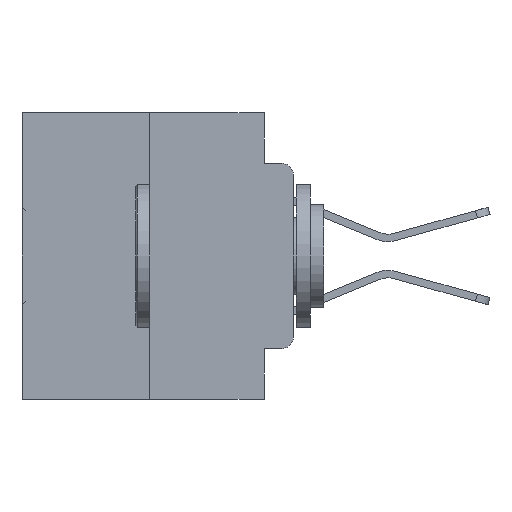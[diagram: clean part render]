
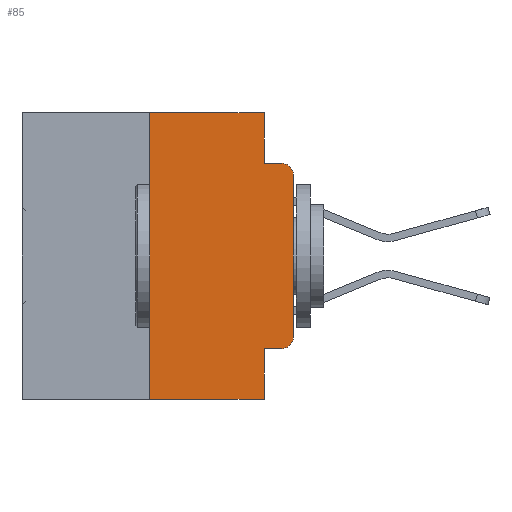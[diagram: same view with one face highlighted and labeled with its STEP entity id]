
A CAD part, left-side view. The second image highlights one B-rep face of the part: STEP entity #85.
In plain terms, the highlighted planar face has unit normal (-1, 0, 0).
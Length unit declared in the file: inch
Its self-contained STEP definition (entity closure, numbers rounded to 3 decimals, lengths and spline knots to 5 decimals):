
#85 = ADVANCED_FACE ( 'NONE', ( #22199 ), #4309, .F. ) ;
#927 = CARTESIAN_POINT ( 'NONE',  ( 0., 0.051, -0.5 ) ) ;
#1116 = AXIS2_PLACEMENT_3D ( 'NONE', #32327, #17435, #2145 ) ;
#1178 = LINE ( 'NONE', #29608, #19971 ) ;
#1871 = DIRECTION ( 'NONE',  ( 0., 0., -1. ) ) ;
#2145 = DIRECTION ( 'NONE',  ( 0., 0., -1. ) ) ;
#2668 = VECTOR ( 'NONE', #17198, 39.37008 ) ;
#2697 = ORIENTED_EDGE ( 'NONE', *, *, #23551, .T. ) ;
#4086 = CARTESIAN_POINT ( 'NONE',  ( 0., 0.473, -0.5 ) ) ;
#4309 = PLANE ( 'NONE',  #28458 ) ;
#4432 = LINE ( 'NONE', #19860, #9673 ) ;
#4903 = EDGE_CURVE ( 'NONE', #10895, #21757, #29985, .T. ) ;
#5461 = VECTOR ( 'NONE', #10900, 39.37008 ) ;
#5634 = CARTESIAN_POINT ( 'NONE',  ( 0., 0.051, -0.4115 ) ) ;
#6263 = LINE ( 'NONE', #5634, #5461 ) ;
#6623 = EDGE_CURVE ( 'NONE', #12689, #10895, #6263, .T. ) ;
#6756 = VECTOR ( 'NONE', #13030, 39.37008 ) ;
#6823 = CIRCLE ( 'NONE', #1116, 0.02 ) ;
#7891 = LINE ( 'NONE', #4086, #14583 ) ;
#8560 = VERTEX_POINT ( 'NONE', #927 ) ;
#8759 = LINE ( 'NONE', #29683, #2668 ) ;
#9404 = DIRECTION ( 'NONE',  ( 0., -1., 0. ) ) ;
#9613 = DIRECTION ( 'NONE',  ( 0., 0., -1. ) ) ;
#9673 = VECTOR ( 'NONE', #9613, 39.37008 ) ;
#9747 = CARTESIAN_POINT ( 'NONE',  ( 0., 0.473, 0. ) ) ;
#10529 = CARTESIAN_POINT ( 'NONE',  ( 0., 0.25, 0. ) ) ;
#10895 = VERTEX_POINT ( 'NONE', #31496 ) ;
#10900 = DIRECTION ( 'NONE',  ( 0., -1., 0. ) ) ;
#10946 = CARTESIAN_POINT ( 'NONE',  ( 0., 0.25, 0. ) ) ;
#11405 = CARTESIAN_POINT ( 'NONE',  ( 0., 0.051, -0.0885 ) ) ;
#11745 = EDGE_CURVE ( 'NONE', #12689, #8560, #4432, .T. ) ;
#12689 = VERTEX_POINT ( 'NONE', #22904 ) ;
#13030 = DIRECTION ( 'NONE',  ( 0., 0., 1. ) ) ;
#13120 = ORIENTED_EDGE ( 'NONE', *, *, #15068, .F. ) ;
#13384 = EDGE_CURVE ( 'NONE', #21767, #18667, #13447, .T. ) ;
#13447 = LINE ( 'NONE', #10529, #6756 ) ;
#13586 = VERTEX_POINT ( 'NONE', #11405 ) ;
#14304 = DIRECTION ( 'NONE',  ( 0., -1., 0. ) ) ;
#14453 = CARTESIAN_POINT ( 'NONE',  ( 0., 0.473, 0. ) ) ;
#14583 = VECTOR ( 'NONE', #14304, 39.37008 ) ;
#15068 = EDGE_CURVE ( 'NONE', #31848, #13586, #1178, .T. ) ;
#15101 = ORIENTED_EDGE ( 'NONE', *, *, #11745, .F. ) ;
#15467 = ORIENTED_EDGE ( 'NONE', *, *, #17006, .F. ) ;
#16682 = ORIENTED_EDGE ( 'NONE', *, *, #6623, .T. ) ;
#16862 = CARTESIAN_POINT ( 'NONE',  ( 0., 0., -0.3915 ) ) ;
#17006 = EDGE_CURVE ( 'NONE', #18667, #31848, #23812, .T. ) ;
#17086 = VECTOR ( 'NONE', #24507, 39.37008 ) ;
#17162 = DIRECTION ( 'NONE',  ( -1., 0., 0. ) ) ;
#17198 = DIRECTION ( 'NONE',  ( 0., 0., 1. ) ) ;
#17435 = DIRECTION ( 'NONE',  ( -1., 0., 0. ) ) ;
#18483 = VERTEX_POINT ( 'NONE', #20222 ) ;
#18667 = VERTEX_POINT ( 'NONE', #10946 ) ;
#18933 = EDGE_CURVE ( 'NONE', #21767, #8560, #7891, .T. ) ;
#19454 = CARTESIAN_POINT ( 'NONE',  ( 0., 0.051, -0.0885 ) ) ;
#19860 = CARTESIAN_POINT ( 'NONE',  ( 0., 0.051, 0. ) ) ;
#19971 = VECTOR ( 'NONE', #22204, 39.37008 ) ;
#20198 = EDGE_CURVE ( 'NONE', #13586, #18483, #29416, .T. ) ;
#20222 = CARTESIAN_POINT ( 'NONE',  ( 0., 0.02, -0.0885 ) ) ;
#21263 = DIRECTION ( 'NONE',  ( 1., 0., 0. ) ) ;
#21757 = VERTEX_POINT ( 'NONE', #16862 ) ;
#21767 = VERTEX_POINT ( 'NONE', #31894 ) ;
#21792 = EDGE_LOOP ( 'NONE', ( #2697, #31109, #25737, #13120, #15467, #25358, #32656, #15101, #16682, #24210 ) ) ;
#21867 = EDGE_CURVE ( 'NONE', #28294, #18483, #6823, .T. ) ;
#22199 = FACE_OUTER_BOUND ( 'NONE', #21792, .T. ) ;
#22204 = DIRECTION ( 'NONE',  ( 0., 0., -1. ) ) ;
#22809 = VECTOR ( 'NONE', #9404, 39.37008 ) ;
#22904 = CARTESIAN_POINT ( 'NONE',  ( 0., 0.051, -0.4115 ) ) ;
#23551 = EDGE_CURVE ( 'NONE', #21757, #28294, #8759, .T. ) ;
#23812 = LINE ( 'NONE', #14453, #17086 ) ;
#24210 = ORIENTED_EDGE ( 'NONE', *, *, #4903, .T. ) ;
#24507 = DIRECTION ( 'NONE',  ( 0., -1., 0. ) ) ;
#25358 = ORIENTED_EDGE ( 'NONE', *, *, #13384, .F. ) ;
#25392 = CARTESIAN_POINT ( 'NONE',  ( 0., 0.051, 0. ) ) ;
#25737 = ORIENTED_EDGE ( 'NONE', *, *, #20198, .F. ) ;
#26678 = DIRECTION ( 'NONE',  ( 0., 0., -1. ) ) ;
#28294 = VERTEX_POINT ( 'NONE', #29577 ) ;
#28458 = AXIS2_PLACEMENT_3D ( 'NONE', #9747, #21263, #26678 ) ;
#29416 = LINE ( 'NONE', #19454, #22809 ) ;
#29577 = CARTESIAN_POINT ( 'NONE',  ( 0., 0., -0.1085 ) ) ;
#29605 = AXIS2_PLACEMENT_3D ( 'NONE', #32063, #17162, #1871 ) ;
#29608 = CARTESIAN_POINT ( 'NONE',  ( 0., 0.051, 0. ) ) ;
#29683 = CARTESIAN_POINT ( 'NONE',  ( 0., 0., 0. ) ) ;
#29985 = CIRCLE ( 'NONE', #29605, 0.02 ) ;
#31109 = ORIENTED_EDGE ( 'NONE', *, *, #21867, .T. ) ;
#31496 = CARTESIAN_POINT ( 'NONE',  ( 0., 0.02, -0.4115 ) ) ;
#31848 = VERTEX_POINT ( 'NONE', #25392 ) ;
#31894 = CARTESIAN_POINT ( 'NONE',  ( 0., 0.25, -0.5 ) ) ;
#32063 = CARTESIAN_POINT ( 'NONE',  ( 0., 0.02, -0.3915 ) ) ;
#32327 = CARTESIAN_POINT ( 'NONE',  ( 0., 0.02, -0.1085 ) ) ;
#32656 = ORIENTED_EDGE ( 'NONE', *, *, #18933, .T. ) ;
